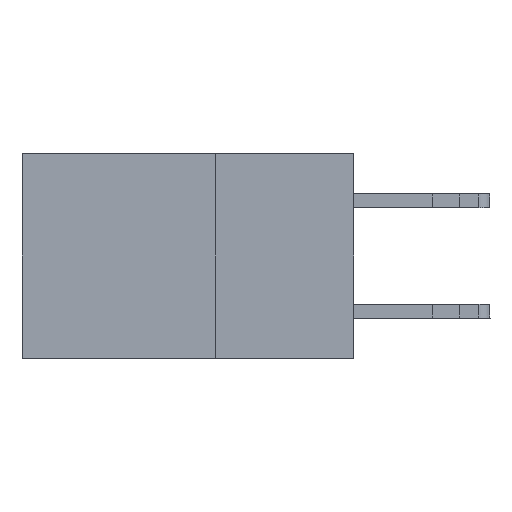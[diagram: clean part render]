
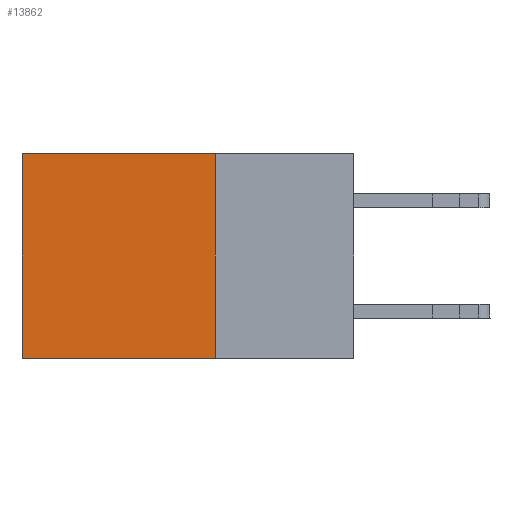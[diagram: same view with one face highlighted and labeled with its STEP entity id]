
A CAD part, left-side view. The second image highlights one B-rep face of the part: STEP entity #13862.
In plain terms, the highlighted planar face has unit normal (-1, 0, 0).
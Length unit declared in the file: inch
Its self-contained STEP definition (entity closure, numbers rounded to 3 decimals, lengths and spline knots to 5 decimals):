
#484 = CARTESIAN_POINT ( 'NONE',  ( 0.2875, 0.6, -0.37 ) ) ;
#741 = CARTESIAN_POINT ( 'NONE',  ( 0.2875, 0.6, 0. ) ) ;
#1315 = CARTESIAN_POINT ( 'NONE',  ( 0.2875, 0.25, 0. ) ) ;
#1705 = ORIENTED_EDGE ( 'NONE', *, *, #25965, .T. ) ;
#2213 = EDGE_LOOP ( 'NONE', ( #1705, #2994, #4612, #28090 ) ) ;
#2629 = VECTOR ( 'NONE', #15673, 39.37008 ) ;
#2994 = ORIENTED_EDGE ( 'NONE', *, *, #9002, .F. ) ;
#3425 = LINE ( 'NONE', #20253, #23025 ) ;
#4612 = ORIENTED_EDGE ( 'NONE', *, *, #26587, .F. ) ;
#5220 = CARTESIAN_POINT ( 'NONE',  ( 0.2875, 0.25, -0.37 ) ) ;
#6179 = CARTESIAN_POINT ( 'NONE',  ( 0.2875, 0.25, -0.37 ) ) ;
#8708 = VERTEX_POINT ( 'NONE', #484 ) ;
#9002 = EDGE_CURVE ( 'NONE', #13623, #8708, #22849, .T. ) ;
#9019 = DIRECTION ( 'NONE',  ( 0., 0., -1. ) ) ;
#9415 = CARTESIAN_POINT ( 'NONE',  ( 0.2875, 0.25, 0. ) ) ;
#10993 = FACE_OUTER_BOUND ( 'NONE', #2213, .T. ) ;
#11059 = VERTEX_POINT ( 'NONE', #1315 ) ;
#12676 = DIRECTION ( 'NONE',  ( 0., 1., 0. ) ) ;
#12799 = DIRECTION ( 'NONE',  ( 0., 0., -1. ) ) ;
#13102 = VECTOR ( 'NONE', #12676, 39.37008 ) ;
#13623 = VERTEX_POINT ( 'NONE', #5220 ) ;
#13862 = ADVANCED_FACE ( 'NONE', ( #10993 ), #26428, .F. ) ;
#15673 = DIRECTION ( 'NONE',  ( 0., 0., -1. ) ) ;
#16937 = VERTEX_POINT ( 'NONE', #741 ) ;
#18719 = EDGE_CURVE ( 'NONE', #11059, #16937, #3425, .T. ) ;
#18854 = CARTESIAN_POINT ( 'NONE',  ( 0.2875, 0.6, 0. ) ) ;
#19366 = AXIS2_PLACEMENT_3D ( 'NONE', #26139, #23994, #12799 ) ;
#20253 = CARTESIAN_POINT ( 'NONE',  ( 0.2875, 0.25, 0. ) ) ;
#20343 = DIRECTION ( 'NONE',  ( 0., 1., 0. ) ) ;
#20467 = VECTOR ( 'NONE', #9019, 39.37008 ) ;
#22849 = LINE ( 'NONE', #6179, #13102 ) ;
#23025 = VECTOR ( 'NONE', #20343, 39.37008 ) ;
#23994 = DIRECTION ( 'NONE',  ( 1., 0., 0. ) ) ;
#25965 = EDGE_CURVE ( 'NONE', #16937, #8708, #26438, .T. ) ;
#26045 = LINE ( 'NONE', #9415, #20467 ) ;
#26139 = CARTESIAN_POINT ( 'NONE',  ( 0.2875, 0.25, 0. ) ) ;
#26428 = PLANE ( 'NONE',  #19366 ) ;
#26438 = LINE ( 'NONE', #18854, #2629 ) ;
#26587 = EDGE_CURVE ( 'NONE', #11059, #13623, #26045, .T. ) ;
#28090 = ORIENTED_EDGE ( 'NONE', *, *, #18719, .T. ) ;
